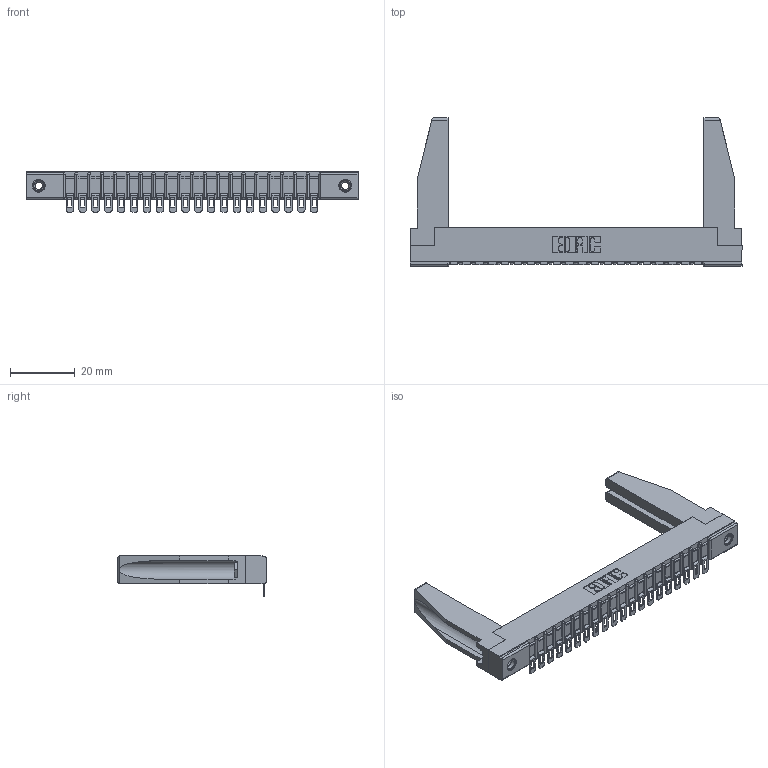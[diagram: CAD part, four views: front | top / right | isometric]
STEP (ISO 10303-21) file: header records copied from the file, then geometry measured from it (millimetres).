
FILE_DESCRIPTION (( 'STEP AP203' ), '1' );
FILE_NAME ('307-020-454-178.STEP', '2020-09-27T03:10:20', ( '' ), ( '' ), 'SwSTEP 2.0', 'SolidWorks 2020', '' );
FILE_SCHEMA (( 'CONFIG_CONTROL_DESIGN' ));
Length unit declared in the file: inch
Products named in the file (5): 307-290-002_554; 307 Part_.156 Dia Mounting Holes; 307-220-078; 345-250-001_345-250-001-102; 307-020-454-178
Assembly tree (25 placements, depth 2):
  307-020-454-178
    307 Part_.156 Dia Mounting Holes
    307-290-002_554  x20
    307-220-078  x2
    345-250-001_345-250-001-102  x2
Bounding box: 102.26 x 45.72 x 12.52 mm (x, y, z)
Volume: 10750.5 mm3; surface area: 16082.1 mm2
Topology: 25 solids, 25 shells, 1889 faces, 5713 edges, 3742 vertices
Faces by surface type: plane 1074, cylinder 757, sphere 42, cone 12, torus 4
Entity records: 23262 total; most frequent: CARTESIAN_POINT 3920, ORIENTED_EDGE 3866, DIRECTION 3781, EDGE_CURVE 1933, VECTOR 1467, LINE 1467, VERTEX_POINT 1254, AXIS2_PLACEMENT_3D 1157
